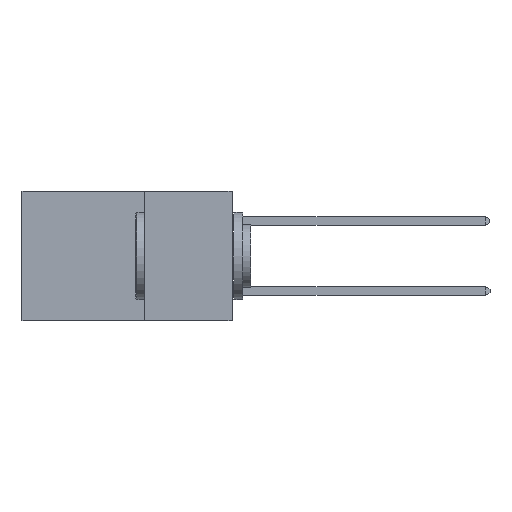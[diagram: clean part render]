
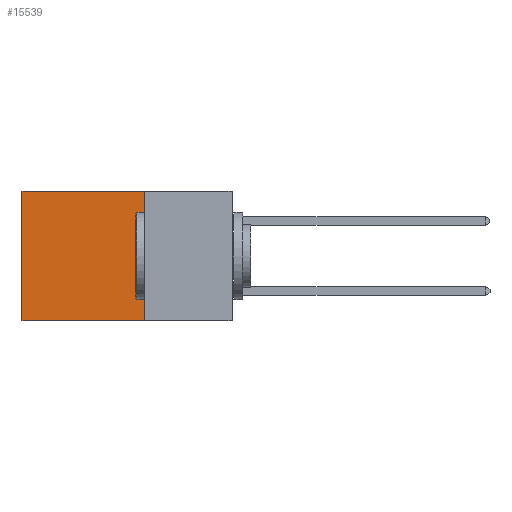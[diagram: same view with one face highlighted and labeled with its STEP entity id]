
A CAD part, left-side view. The second image highlights one B-rep face of the part: STEP entity #15539.
In plain terms, the highlighted planar face has unit normal (-1, 0, 0).
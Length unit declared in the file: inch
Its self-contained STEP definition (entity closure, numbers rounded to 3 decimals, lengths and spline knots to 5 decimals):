
#113 = EDGE_LOOP ( 'NONE', ( #18051, #11627, #14784, #391 ) ) ;
#391 = ORIENTED_EDGE ( 'NONE', *, *, #8362, .T. ) ;
#1116 = DIRECTION ( 'NONE',  ( 0., 0., -1. ) ) ;
#2004 = PLANE ( 'NONE',  #15759 ) ;
#3488 = VERTEX_POINT ( 'NONE', #13104 ) ;
#4565 = CARTESIAN_POINT ( 'NONE',  ( 0.2875, 0.25, -0.37 ) ) ;
#4694 = LINE ( 'NONE', #18615, #8268 ) ;
#5134 = DIRECTION ( 'NONE',  ( 0., 0., -1. ) ) ;
#5777 = EDGE_CURVE ( 'NONE', #9198, #3488, #18404, .T. ) ;
#6593 = CARTESIAN_POINT ( 'NONE',  ( 0.2875, 0.25, 0. ) ) ;
#7909 = DIRECTION ( 'NONE',  ( 0., 1., 0. ) ) ;
#8268 = VECTOR ( 'NONE', #7909, 39.37008 ) ;
#8362 = EDGE_CURVE ( 'NONE', #11388, #8931, #4694, .T. ) ;
#8931 = VERTEX_POINT ( 'NONE', #13680 ) ;
#9198 = VERTEX_POINT ( 'NONE', #13070 ) ;
#9693 = FACE_OUTER_BOUND ( 'NONE', #113, .T. ) ;
#9811 = LINE ( 'NONE', #14157, #17943 ) ;
#10612 = VECTOR ( 'NONE', #1116, 39.37008 ) ;
#10696 = DIRECTION ( 'NONE',  ( 0., 1., 0. ) ) ;
#11388 = VERTEX_POINT ( 'NONE', #17237 ) ;
#11627 = ORIENTED_EDGE ( 'NONE', *, *, #5777, .F. ) ;
#13070 = CARTESIAN_POINT ( 'NONE',  ( 0.2875, 0.25, -0.37 ) ) ;
#13104 = CARTESIAN_POINT ( 'NONE',  ( 0.2875, 0.6, -0.37 ) ) ;
#13415 = CARTESIAN_POINT ( 'NONE',  ( 0.2875, 0.25, 0. ) ) ;
#13680 = CARTESIAN_POINT ( 'NONE',  ( 0.2875, 0.6, 0. ) ) ;
#14157 = CARTESIAN_POINT ( 'NONE',  ( 0.2875, 0.6, 0. ) ) ;
#14229 = DIRECTION ( 'NONE',  ( 1., 0., 0. ) ) ;
#14784 = ORIENTED_EDGE ( 'NONE', *, *, #17739, .F. ) ;
#15539 = ADVANCED_FACE ( 'NONE', ( #9693 ), #2004, .F. ) ;
#15667 = DIRECTION ( 'NONE',  ( 0., 0., -1. ) ) ;
#15759 = AXIS2_PLACEMENT_3D ( 'NONE', #6593, #14229, #5134 ) ;
#17237 = CARTESIAN_POINT ( 'NONE',  ( 0.2875, 0.25, 0. ) ) ;
#17739 = EDGE_CURVE ( 'NONE', #11388, #9198, #19264, .T. ) ;
#17943 = VECTOR ( 'NONE', #15667, 39.37008 ) ;
#18051 = ORIENTED_EDGE ( 'NONE', *, *, #19857, .T. ) ;
#18211 = VECTOR ( 'NONE', #10696, 39.37008 ) ;
#18404 = LINE ( 'NONE', #4565, #18211 ) ;
#18615 = CARTESIAN_POINT ( 'NONE',  ( 0.2875, 0.25, 0. ) ) ;
#19264 = LINE ( 'NONE', #13415, #10612 ) ;
#19857 = EDGE_CURVE ( 'NONE', #8931, #3488, #9811, .T. ) ;
